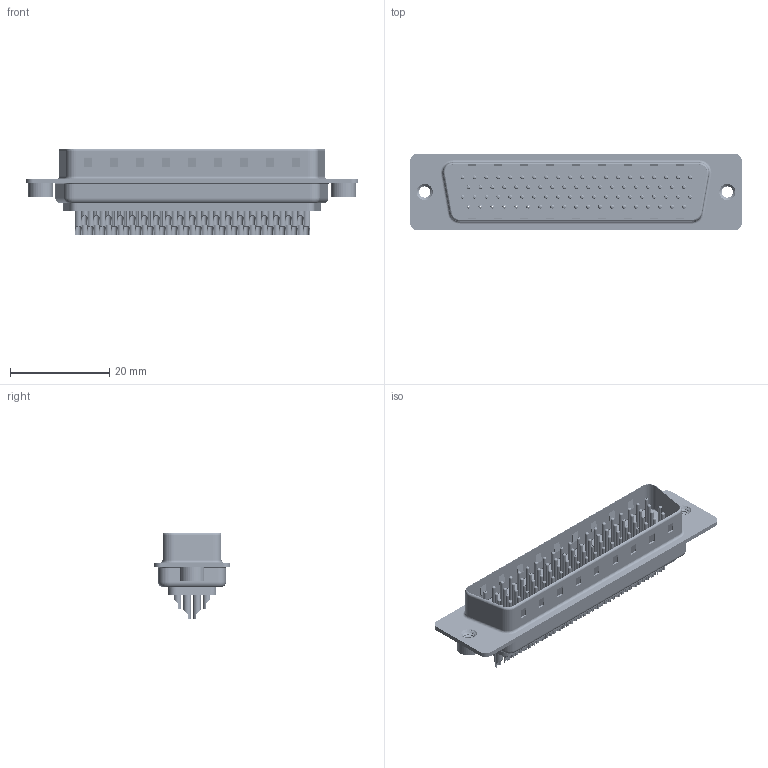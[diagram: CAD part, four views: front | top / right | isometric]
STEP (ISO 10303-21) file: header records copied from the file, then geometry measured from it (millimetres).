
FILE_DESCRIPTION (( 'STEP AP203' ), '1' );
FILE_NAME ('637-078-232-042.STEP', '2020-07-18T05:21:24', ( '' ), ( '' ), 'SwSTEP 2.0', 'SolidWorks 2020', '' );
FILE_SCHEMA (( 'CONFIG_CONTROL_DESIGN' ));
Length unit declared in the file: millimetre
Products named in the file (9): 637 Housing_78 Contacts; 637 Contact Row 78_32; 637-078-232-042; 637 Shell Rear_78 Contacts; 637 Shell Front_78 Contacts; 637 Contact Row 3_32; 637 4-40 Threaded Rivet; 637 Contact Row 1_32(78); 637 Contact Row 2_32(78)
Assembly tree (83 placements, depth 2):
  637-078-232-042
    637 Housing_78 Contacts
    637 Shell Front_78 Contacts
    637 Shell Rear_78 Contacts
    637 Contact Row 1_32(78)  x19
    637 Contact Row 2_32(78)  x20
    637 Contact Row 3_32  x19
    637 Contact Row 78_32  x20
    637 4-40 Threaded Rivet  x2
Bounding box: 67 x 15.4 x 17.55 mm (x, y, z)
Volume: 4434.8 mm3; surface area: 16779.9 mm2
Topology: 83 solids, 83 shells, 5404 faces, 13849 edges, 8778 vertices
Faces by surface type: cylinder 2403, torus 1688, plane 1295, cone 12, bspline 6
Entity records: 41574 total; most frequent: CARTESIAN_POINT 7901, DIRECTION 7058, ORIENTED_EDGE 5928, EDGE_CURVE 2964, AXIS2_PLACEMENT_3D 2879, VERTEX_POINT 1918, EDGE_LOOP 1598, CIRCLE 1569
